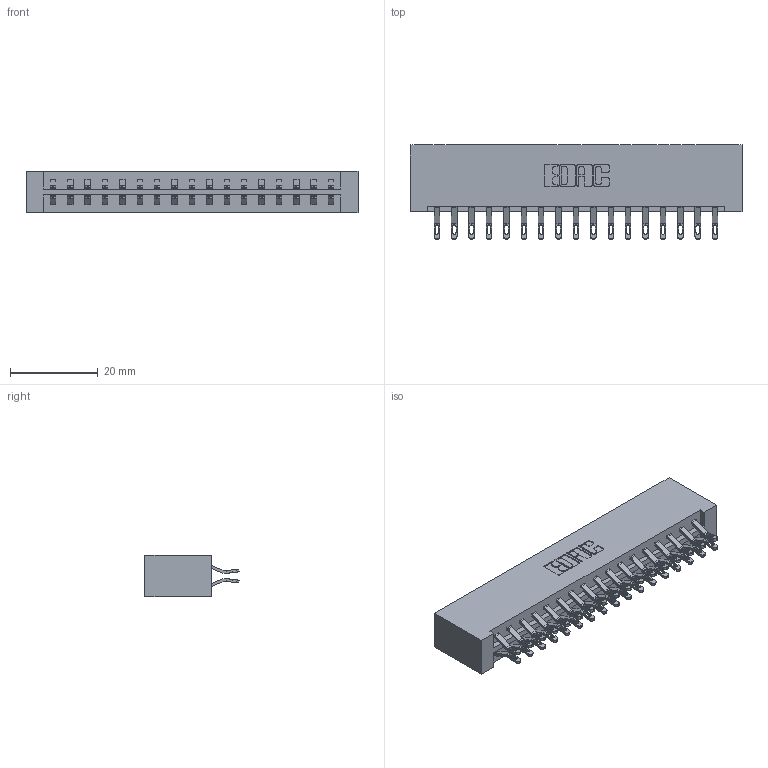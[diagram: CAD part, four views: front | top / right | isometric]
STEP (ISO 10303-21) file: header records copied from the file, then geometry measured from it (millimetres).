
FILE_DESCRIPTION (( 'STEP AP203' ), '1' );
FILE_NAME ('833-034-555-201.STEP', '2020-06-02T23:05:09', ( '' ), ( '' ), 'SwSTEP 2.0', 'SolidWorks 2020', '' );
FILE_SCHEMA (( 'CONFIG_CONTROL_DESIGN' ));
Length unit declared in the file: inch
Products named in the file (3): 833 Part_Lugless; 345-292-001_555 Tail; 833-034-555-201
Assembly tree (35 placements, depth 2):
  833-034-555-201
    833 Part_Lugless
    345-292-001_555 Tail  x34
Bounding box: 75.62 x 21.47 x 9.4 mm (x, y, z)
Volume: 8217 mm3; surface area: 9839.1 mm2
Topology: 35 solids, 35 shells, 2078 faces, 6509 edges, 4338 vertices
Faces by surface type: plane 1222, cylinder 856
Entity records: 14219 total; most frequent: CARTESIAN_POINT 2420, ORIENTED_EDGE 2326, DIRECTION 2075, EDGE_CURVE 1163, LINE 1023, VECTOR 1023, VERTEX_POINT 774, AXIS2_PLACEMENT_3D 526
